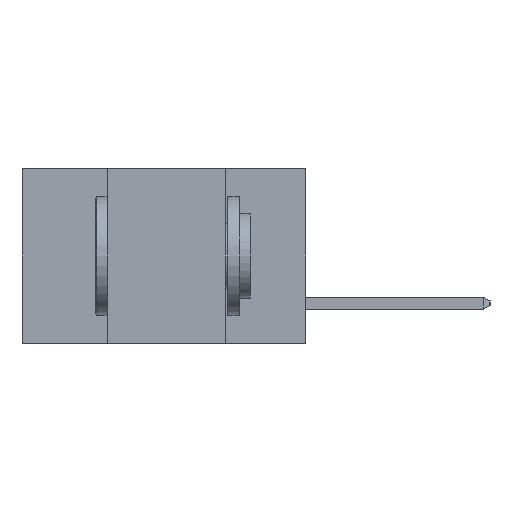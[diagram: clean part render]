
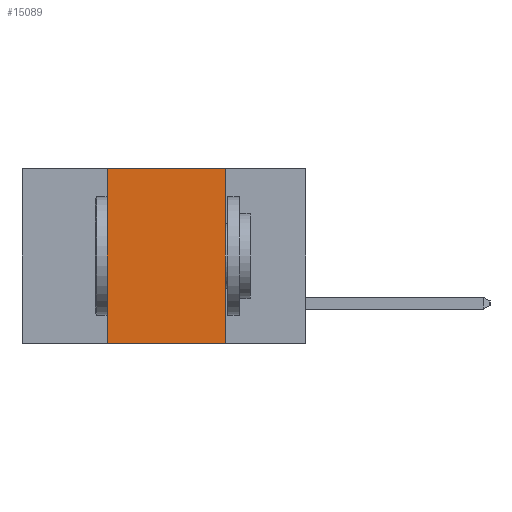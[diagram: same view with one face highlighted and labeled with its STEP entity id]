
A CAD part, left-side view. The second image highlights one B-rep face of the part: STEP entity #15089.
In plain terms, the highlighted planar face has unit normal (-1, 0, 0).
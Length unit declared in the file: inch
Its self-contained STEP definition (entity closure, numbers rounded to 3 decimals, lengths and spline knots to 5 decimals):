
#165 = EDGE_CURVE ( 'NONE', #12603, #10902, #10607, .T. ) ;
#179 = PLANE ( 'NONE',  #13397 ) ;
#298 = VECTOR ( 'NONE', #5666, 39.37008 ) ;
#999 = EDGE_CURVE ( 'NONE', #15081, #3164, #3585, .T. ) ;
#1163 = ORIENTED_EDGE ( 'NONE', *, *, #999, .F. ) ;
#1353 = CARTESIAN_POINT ( 'NONE',  ( 0., 0.17, -0.37 ) ) ;
#1438 = DIRECTION ( 'NONE',  ( 0., -1., 0. ) ) ;
#1537 = ORIENTED_EDGE ( 'NONE', *, *, #2666, .F. ) ;
#1683 = FACE_OUTER_BOUND ( 'NONE', #10177, .T. ) ;
#1783 = VECTOR ( 'NONE', #1438, 39.37008 ) ;
#1921 = ORIENTED_EDGE ( 'NONE', *, *, #165, .F. ) ;
#2643 = CARTESIAN_POINT ( 'NONE',  ( 0., 0.6, 0. ) ) ;
#2666 = EDGE_CURVE ( 'NONE', #3164, #12603, #5051, .T. ) ;
#3164 = VERTEX_POINT ( 'NONE', #9360 ) ;
#3585 = LINE ( 'NONE', #5515, #298 ) ;
#3917 = DIRECTION ( 'NONE',  ( 0., 0., -1. ) ) ;
#4107 = LINE ( 'NONE', #15921, #10302 ) ;
#5051 = LINE ( 'NONE', #14570, #1783 ) ;
#5515 = CARTESIAN_POINT ( 'NONE',  ( 0., 0.42, 0. ) ) ;
#5666 = DIRECTION ( 'NONE',  ( 0., 0., 1. ) ) ;
#7446 = CARTESIAN_POINT ( 'NONE',  ( 0., 0.17, 0. ) ) ;
#9360 = CARTESIAN_POINT ( 'NONE',  ( 0., 0.42, 0. ) ) ;
#9586 = CARTESIAN_POINT ( 'NONE',  ( 0., 0.17, 0. ) ) ;
#9694 = DIRECTION ( 'NONE',  ( 0., -1., 0. ) ) ;
#9861 = ORIENTED_EDGE ( 'NONE', *, *, #10111, .T. ) ;
#10111 = EDGE_CURVE ( 'NONE', #15081, #10902, #4107, .T. ) ;
#10177 = EDGE_LOOP ( 'NONE', ( #1921, #1537, #1163, #9861 ) ) ;
#10302 = VECTOR ( 'NONE', #9694, 39.37008 ) ;
#10607 = LINE ( 'NONE', #7446, #13132 ) ;
#10902 = VERTEX_POINT ( 'NONE', #1353 ) ;
#11338 = DIRECTION ( 'NONE',  ( 1., 0., 0. ) ) ;
#12603 = VERTEX_POINT ( 'NONE', #9586 ) ;
#13132 = VECTOR ( 'NONE', #14501, 39.37008 ) ;
#13397 = AXIS2_PLACEMENT_3D ( 'NONE', #2643, #11338, #3917 ) ;
#14501 = DIRECTION ( 'NONE',  ( 0., 0., -1. ) ) ;
#14570 = CARTESIAN_POINT ( 'NONE',  ( 0., 0.6, 0. ) ) ;
#15011 = CARTESIAN_POINT ( 'NONE',  ( 0., 0.42, -0.37 ) ) ;
#15081 = VERTEX_POINT ( 'NONE', #15011 ) ;
#15089 = ADVANCED_FACE ( 'NONE', ( #1683 ), #179, .F. ) ;
#15921 = CARTESIAN_POINT ( 'NONE',  ( 0., 0.6, -0.37 ) ) ;
